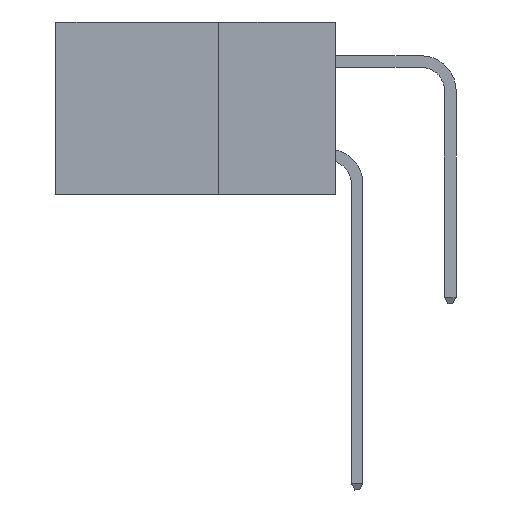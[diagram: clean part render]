
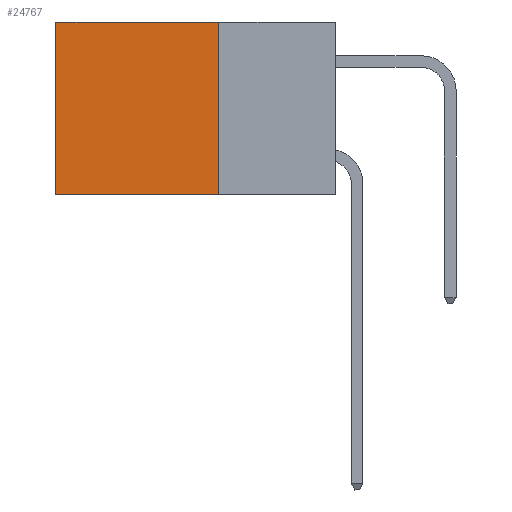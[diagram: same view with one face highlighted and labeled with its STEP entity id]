
A CAD part, left-side view. The second image highlights one B-rep face of the part: STEP entity #24767.
In plain terms, the highlighted planar face has unit normal (-1, 0, 0).
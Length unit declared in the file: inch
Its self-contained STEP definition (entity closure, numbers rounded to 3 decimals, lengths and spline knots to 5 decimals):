
#2595 = ORIENTED_EDGE ( 'NONE', *, *, #20030, .F. ) ;
#3250 = ORIENTED_EDGE ( 'NONE', *, *, #29706, .T. ) ;
#4763 = PLANE ( 'NONE',  #9453 ) ;
#5373 = VERTEX_POINT ( 'NONE', #32327 ) ;
#7846 = CARTESIAN_POINT ( 'NONE',  ( 0.2875, 0.25, 0. ) ) ;
#9453 = AXIS2_PLACEMENT_3D ( 'NONE', #7846, #29009, #10919 ) ;
#10919 = DIRECTION ( 'NONE',  ( 0., 0., -1. ) ) ;
#10932 = DIRECTION ( 'NONE',  ( 0., 1., 0. ) ) ;
#13690 = VECTOR ( 'NONE', #19010, 39.37008 ) ;
#15588 = VECTOR ( 'NONE', #30800, 39.37008 ) ;
#15628 = CARTESIAN_POINT ( 'NONE',  ( 0.2875, 0.25, -0.37 ) ) ;
#15775 = VERTEX_POINT ( 'NONE', #28309 ) ;
#16524 = LINE ( 'NONE', #18668, #15588 ) ;
#18023 = CARTESIAN_POINT ( 'NONE',  ( 0.2875, 0.25, 0. ) ) ;
#18219 = EDGE_CURVE ( 'NONE', #26841, #26971, #21735, .T. ) ;
#18623 = VECTOR ( 'NONE', #10932, 39.37008 ) ;
#18668 = CARTESIAN_POINT ( 'NONE',  ( 0.2875, 0.25, -0.37 ) ) ;
#19010 = DIRECTION ( 'NONE',  ( 0., 0., -1. ) ) ;
#20030 = EDGE_CURVE ( 'NONE', #26971, #15775, #16524, .T. ) ;
#21735 = LINE ( 'NONE', #31148, #13690 ) ;
#22942 = CARTESIAN_POINT ( 'NONE',  ( 0.2875, 0.25, 0. ) ) ;
#24569 = VECTOR ( 'NONE', #36375, 39.37008 ) ;
#24767 = ADVANCED_FACE ( 'NONE', ( #33205 ), #4763, .F. ) ;
#25047 = EDGE_LOOP ( 'NONE', ( #3250, #2595, #31589, #35569 ) ) ;
#25505 = LINE ( 'NONE', #33380, #24569 ) ;
#26617 = LINE ( 'NONE', #22942, #18623 ) ;
#26841 = VERTEX_POINT ( 'NONE', #18023 ) ;
#26971 = VERTEX_POINT ( 'NONE', #15628 ) ;
#28309 = CARTESIAN_POINT ( 'NONE',  ( 0.2875, 0.6, -0.37 ) ) ;
#29009 = DIRECTION ( 'NONE',  ( 1., 0., 0. ) ) ;
#29706 = EDGE_CURVE ( 'NONE', #5373, #15775, #25505, .T. ) ;
#30800 = DIRECTION ( 'NONE',  ( 0., 1., 0. ) ) ;
#31148 = CARTESIAN_POINT ( 'NONE',  ( 0.2875, 0.25, 0. ) ) ;
#31589 = ORIENTED_EDGE ( 'NONE', *, *, #18219, .F. ) ;
#32327 = CARTESIAN_POINT ( 'NONE',  ( 0.2875, 0.6, 0. ) ) ;
#33205 = FACE_OUTER_BOUND ( 'NONE', #25047, .T. ) ;
#33380 = CARTESIAN_POINT ( 'NONE',  ( 0.2875, 0.6, 0. ) ) ;
#35569 = ORIENTED_EDGE ( 'NONE', *, *, #38556, .T. ) ;
#36375 = DIRECTION ( 'NONE',  ( 0., 0., -1. ) ) ;
#38556 = EDGE_CURVE ( 'NONE', #26841, #5373, #26617, .T. ) ;
